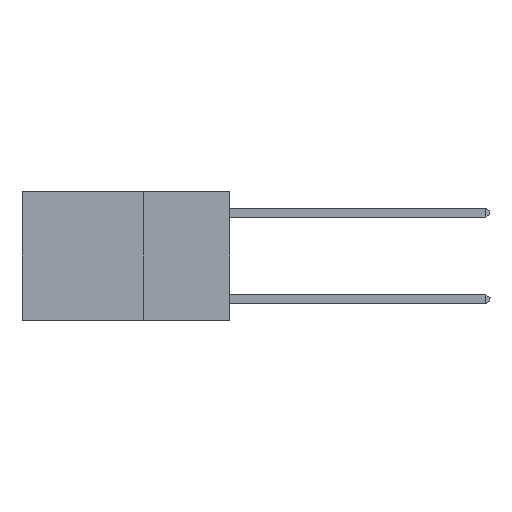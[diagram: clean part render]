
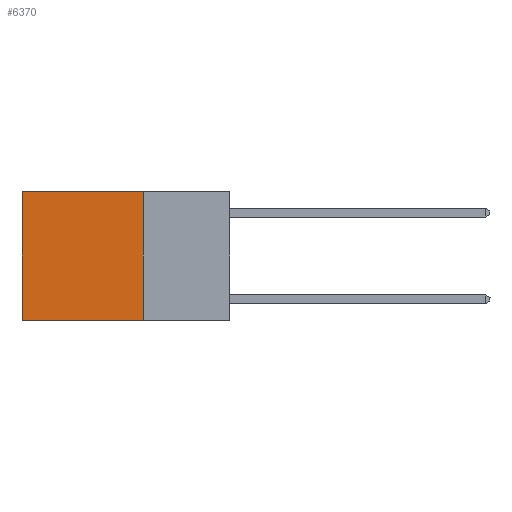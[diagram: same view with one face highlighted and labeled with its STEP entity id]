
A CAD part, left-side view. The second image highlights one B-rep face of the part: STEP entity #6370.
In plain terms, the highlighted planar face has unit normal (-1, 0, 0).
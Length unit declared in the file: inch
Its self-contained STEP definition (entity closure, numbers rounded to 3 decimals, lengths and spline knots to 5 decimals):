
#25 = CARTESIAN_POINT ( 'NONE',  ( 0.2625, 0.6, 0. ) ) ;
#231 = CARTESIAN_POINT ( 'NONE',  ( 0.2625, 0.25, 0. ) ) ;
#1099 = ORIENTED_EDGE ( 'NONE', *, *, #17326, .T. ) ;
#1183 = CARTESIAN_POINT ( 'NONE',  ( 0.2625, 0.6, -0.37 ) ) ;
#2330 = DIRECTION ( 'NONE',  ( 0., 0., -1. ) ) ;
#2772 = VECTOR ( 'NONE', #9533, 39.37008 ) ;
#3881 = ORIENTED_EDGE ( 'NONE', *, *, #11349, .F. ) ;
#4123 = VERTEX_POINT ( 'NONE', #16509 ) ;
#4415 = VECTOR ( 'NONE', #13755, 39.37008 ) ;
#4753 = LINE ( 'NONE', #15727, #24097 ) ;
#4938 = VERTEX_POINT ( 'NONE', #25 ) ;
#5552 = LINE ( 'NONE', #23582, #4415 ) ;
#6044 = EDGE_CURVE ( 'NONE', #4123, #7338, #13607, .T. ) ;
#6370 = ADVANCED_FACE ( 'NONE', ( #16666 ), #12543, .F. ) ;
#7338 = VERTEX_POINT ( 'NONE', #1183 ) ;
#7482 = CARTESIAN_POINT ( 'NONE',  ( 0.2625, 0.25, -0.37 ) ) ;
#7619 = LINE ( 'NONE', #8318, #18253 ) ;
#8318 = CARTESIAN_POINT ( 'NONE',  ( 0.2625, 0.6, 0. ) ) ;
#8425 = EDGE_LOOP ( 'NONE', ( #1099, #15829, #3881, #8639 ) ) ;
#8639 = ORIENTED_EDGE ( 'NONE', *, *, #14617, .T. ) ;
#9533 = DIRECTION ( 'NONE',  ( 0., 1., 0. ) ) ;
#11349 = EDGE_CURVE ( 'NONE', #23969, #4123, #5552, .T. ) ;
#11557 = AXIS2_PLACEMENT_3D ( 'NONE', #231, #14540, #2330 ) ;
#12543 = PLANE ( 'NONE',  #11557 ) ;
#13607 = LINE ( 'NONE', #7482, #2772 ) ;
#13755 = DIRECTION ( 'NONE',  ( 0., 0., -1. ) ) ;
#14540 = DIRECTION ( 'NONE',  ( 1., 0., 0. ) ) ;
#14617 = EDGE_CURVE ( 'NONE', #23969, #4938, #4753, .T. ) ;
#15727 = CARTESIAN_POINT ( 'NONE',  ( 0.2625, 0.25, 0. ) ) ;
#15829 = ORIENTED_EDGE ( 'NONE', *, *, #6044, .F. ) ;
#16345 = CARTESIAN_POINT ( 'NONE',  ( 0.2625, 0.25, 0. ) ) ;
#16509 = CARTESIAN_POINT ( 'NONE',  ( 0.2625, 0.25, -0.37 ) ) ;
#16666 = FACE_OUTER_BOUND ( 'NONE', #8425, .T. ) ;
#17326 = EDGE_CURVE ( 'NONE', #4938, #7338, #7619, .T. ) ;
#17700 = DIRECTION ( 'NONE',  ( 0., 1., 0. ) ) ;
#18253 = VECTOR ( 'NONE', #20255, 39.37008 ) ;
#20255 = DIRECTION ( 'NONE',  ( 0., 0., -1. ) ) ;
#23582 = CARTESIAN_POINT ( 'NONE',  ( 0.2625, 0.25, 0. ) ) ;
#23969 = VERTEX_POINT ( 'NONE', #16345 ) ;
#24097 = VECTOR ( 'NONE', #17700, 39.37008 ) ;
